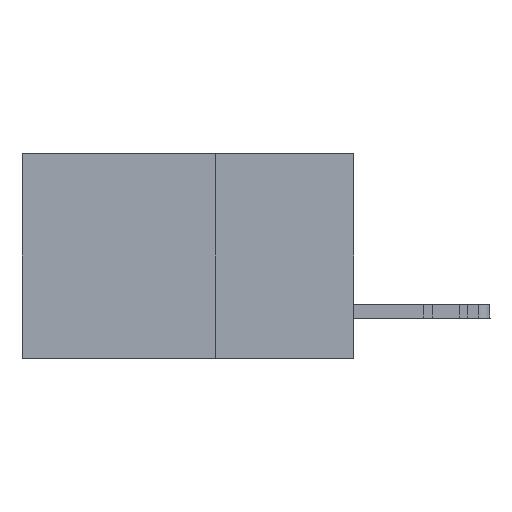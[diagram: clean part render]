
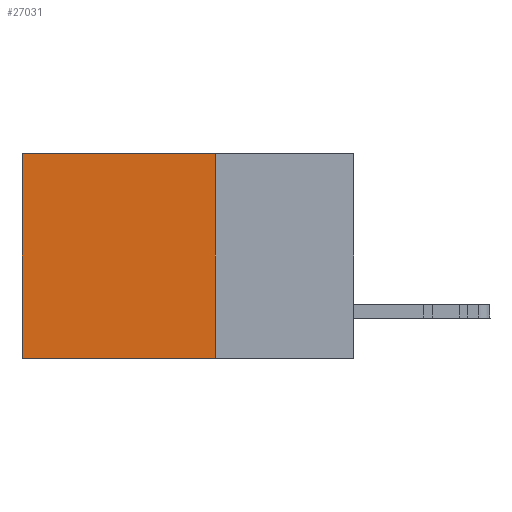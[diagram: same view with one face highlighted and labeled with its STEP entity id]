
A CAD part, left-side view. The second image highlights one B-rep face of the part: STEP entity #27031.
In plain terms, the highlighted planar face has unit normal (-1, 0, 0).
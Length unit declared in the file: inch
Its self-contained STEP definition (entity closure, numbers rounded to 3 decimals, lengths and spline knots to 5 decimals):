
#247 = CARTESIAN_POINT ( 'NONE',  ( 0.2875, 0.6, 0. ) ) ;
#1538 = LINE ( 'NONE', #34603, #12395 ) ;
#2556 = PLANE ( 'NONE',  #37864 ) ;
#3064 = DIRECTION ( 'NONE',  ( 0., 0., -1. ) ) ;
#3281 = VERTEX_POINT ( 'NONE', #25639 ) ;
#4815 = DIRECTION ( 'NONE',  ( 0., 0., -1. ) ) ;
#8289 = ORIENTED_EDGE ( 'NONE', *, *, #38961, .F. ) ;
#9859 = CARTESIAN_POINT ( 'NONE',  ( 0.2875, 0.25, 0. ) ) ;
#10535 = EDGE_CURVE ( 'NONE', #22795, #44428, #17181, .T. ) ;
#12395 = VECTOR ( 'NONE', #46918, 39.37008 ) ;
#14118 = CARTESIAN_POINT ( 'NONE',  ( 0.2875, 0.25, -0.37 ) ) ;
#15516 = ORIENTED_EDGE ( 'NONE', *, *, #25530, .T. ) ;
#16426 = DIRECTION ( 'NONE',  ( 0., 0., -1. ) ) ;
#17181 = LINE ( 'NONE', #32610, #49151 ) ;
#21628 = LINE ( 'NONE', #9859, #49358 ) ;
#21978 = CARTESIAN_POINT ( 'NONE',  ( 0.2875, 0.25, 0. ) ) ;
#22795 = VERTEX_POINT ( 'NONE', #14118 ) ;
#24377 = DIRECTION ( 'NONE',  ( 0., 1., 0. ) ) ;
#25530 = EDGE_CURVE ( 'NONE', #44643, #44428, #28020, .T. ) ;
#25639 = CARTESIAN_POINT ( 'NONE',  ( 0.2875, 0.25, 0. ) ) ;
#27031 = ADVANCED_FACE ( 'NONE', ( #36572 ), #2556, .F. ) ;
#28020 = LINE ( 'NONE', #47318, #49228 ) ;
#28679 = EDGE_LOOP ( 'NONE', ( #15516, #36680, #8289, #34968 ) ) ;
#32332 = EDGE_CURVE ( 'NONE', #3281, #44643, #1538, .T. ) ;
#32610 = CARTESIAN_POINT ( 'NONE',  ( 0.2875, 0.25, -0.37 ) ) ;
#34603 = CARTESIAN_POINT ( 'NONE',  ( 0.2875, 0.25, 0. ) ) ;
#34968 = ORIENTED_EDGE ( 'NONE', *, *, #32332, .T. ) ;
#36572 = FACE_OUTER_BOUND ( 'NONE', #28679, .T. ) ;
#36680 = ORIENTED_EDGE ( 'NONE', *, *, #10535, .F. ) ;
#37819 = DIRECTION ( 'NONE',  ( 1., 0., 0. ) ) ;
#37864 = AXIS2_PLACEMENT_3D ( 'NONE', #21978, #37819, #3064 ) ;
#38961 = EDGE_CURVE ( 'NONE', #3281, #22795, #21628, .T. ) ;
#41810 = CARTESIAN_POINT ( 'NONE',  ( 0.2875, 0.6, -0.37 ) ) ;
#44428 = VERTEX_POINT ( 'NONE', #41810 ) ;
#44643 = VERTEX_POINT ( 'NONE', #247 ) ;
#46918 = DIRECTION ( 'NONE',  ( 0., 1., 0. ) ) ;
#47318 = CARTESIAN_POINT ( 'NONE',  ( 0.2875, 0.6, 0. ) ) ;
#49151 = VECTOR ( 'NONE', #24377, 39.37008 ) ;
#49228 = VECTOR ( 'NONE', #4815, 39.37008 ) ;
#49358 = VECTOR ( 'NONE', #16426, 39.37008 ) ;
